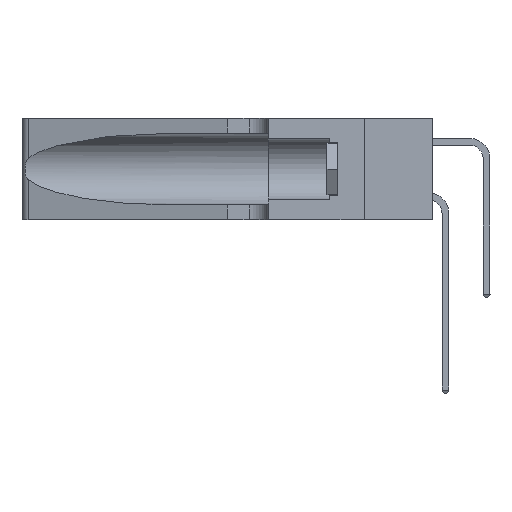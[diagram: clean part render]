
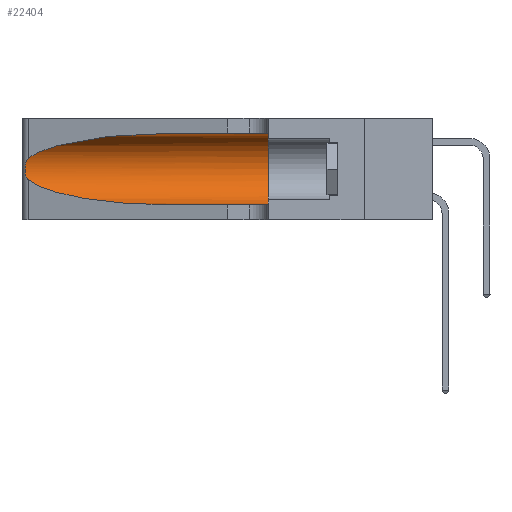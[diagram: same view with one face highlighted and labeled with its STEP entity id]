
A CAD part, left-side view. The second image highlights one B-rep face of the part: STEP entity #22404.
In plain terms, the highlighted cylindrical face has radius 3.308 mm (diameter 6.617 mm), a partial arc.
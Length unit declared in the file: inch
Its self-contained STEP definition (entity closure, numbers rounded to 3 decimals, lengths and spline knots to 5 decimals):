
#480 = CARTESIAN_POINT ( 'NONE',  ( 0.1305, 0.35, 0.05475 ) ) ;
#1663 = VECTOR ( 'NONE', #10198, 39.37008 ) ;
#1909 = CARTESIAN_POINT ( 'NONE',  ( 0.1305, 0.72297, 0.31525 ) ) ;
#1975 = CARTESIAN_POINT ( 'NONE',  ( 0.25555, 1.22993, 0.14849 ) ) ;
#2083 = ORIENTED_EDGE ( 'NONE', *, *, #28961, .T. ) ;
#4200 = CARTESIAN_POINT ( 'NONE',  ( 0.1305, 1.61858, 0.05475 ) ) ;
#4732 =( BOUNDED_CURVE ( )  B_SPLINE_CURVE ( 3, ( #27735, #27615, #33720, #15820 ),
 .UNSPECIFIED., .F., .T. ) 
 B_SPLINE_CURVE_WITH_KNOTS ( ( 4, 4 ),
 ( 1.5708, 2.84003 ),
 .UNSPECIFIED. ) 
 CURVE ( )  GEOMETRIC_REPRESENTATION_ITEM ( )  RATIONAL_B_SPLINE_CURVE ( ( 1., 0.87, 0.87, 1. ) ) 
 REPRESENTATION_ITEM ( '' )  );
#4814 = EDGE_CURVE ( 'NONE', #10529, #27757, #31335, .T. ) ;
#4888 = CARTESIAN_POINT ( 'NONE',  ( 0.25555, 1.22994, 0.2215 ) ) ;
#5431 = CARTESIAN_POINT ( 'NONE',  ( 0.25487, 1.22718, 0.14631 ) ) ;
#5658 = VERTEX_POINT ( 'NONE', #14777 ) ;
#5668 = CYLINDRICAL_SURFACE ( 'NONE', #28201, 0.13025 ) ;
#6494 = CARTESIAN_POINT ( 'NONE',  ( 0.1305, 1.61858, 0.185 ) ) ;
#7881 = CARTESIAN_POINT ( 'NONE',  ( 0.25787, 1.23484, 0.2124 ) ) ;
#9592 = CARTESIAN_POINT ( 'NONE',  ( 0.25487, 1.22718, 0.14631 ) ) ;
#9637 = LINE ( 'NONE', #4200, #1663 ) ;
#10198 = DIRECTION ( 'NONE',  ( 0., -1., 0. ) ) ;
#10529 = VERTEX_POINT ( 'NONE', #23702 ) ;
#10869 = CARTESIAN_POINT ( 'NONE',  ( 0.26018, 1.23835, 0.19895 ) ) ;
#11969 = DIRECTION ( 'NONE',  ( 0., -1., 0. ) ) ;
#13504 = DIRECTION ( 'NONE',  ( 0., 1., 0. ) ) ;
#13887 = CARTESIAN_POINT ( 'NONE',  ( 0.26075, 1.23896, 0.178 ) ) ;
#14024 = EDGE_CURVE ( 'NONE', #27757, #5658, #28487, .T. ) ;
#14453 = CARTESIAN_POINT ( 'NONE',  ( 0.1305, 0.72297, 0.05475 ) ) ;
#14777 = CARTESIAN_POINT ( 'NONE',  ( 0.1305, 0.72297, 0.05475 ) ) ;
#15820 = CARTESIAN_POINT ( 'NONE',  ( 0.25487, 1.22718, 0.22369 ) ) ;
#16603 = CARTESIAN_POINT ( 'NONE',  ( 0.1305, 0.35, 0.31525 ) ) ;
#16922 = CARTESIAN_POINT ( 'NONE',  ( 0.25856, 1.23593, 0.16098 ) ) ;
#17282 = VERTEX_POINT ( 'NONE', #1909 ) ;
#17672 = ORIENTED_EDGE ( 'NONE', *, *, #33002, .F. ) ;
#18349 = VECTOR ( 'NONE', #11969, 39.37008 ) ;
#18888 = ORIENTED_EDGE ( 'NONE', *, *, #14024, .T. ) ;
#19963 = CARTESIAN_POINT ( 'NONE',  ( 0.25639, 1.23186, 0.15144 ) ) ;
#22276 = EDGE_CURVE ( 'NONE', #17282, #31079, #35158, .T. ) ;
#22404 = ADVANCED_FACE ( 'NONE', ( #22557 ), #5668, .F. ) ;
#22557 = FACE_OUTER_BOUND ( 'NONE', #38370, .T. ) ;
#22687 = VERTEX_POINT ( 'NONE', #480 ) ;
#22972 = CARTESIAN_POINT ( 'NONE',  ( 0.25487, 1.22718, 0.14631 ) ) ;
#23365 = CARTESIAN_POINT ( 'NONE',  ( 0.2373, 1.15595, 0.08982 ) ) ;
#23702 = CARTESIAN_POINT ( 'NONE',  ( 0.25487, 1.22718, 0.22369 ) ) ;
#25795 = CARTESIAN_POINT ( 'NONE',  ( 0.25639, 1.23184, 0.21858 ) ) ;
#27376 = ORIENTED_EDGE ( 'NONE', *, *, #36530, .T. ) ;
#27615 = CARTESIAN_POINT ( 'NONE',  ( 0.18966, 0.96281, 0.31525 ) ) ;
#27735 = CARTESIAN_POINT ( 'NONE',  ( 0.1305, 0.72297, 0.31525 ) ) ;
#27757 = VERTEX_POINT ( 'NONE', #9592 ) ;
#28128 = ORIENTED_EDGE ( 'NONE', *, *, #22276, .F. ) ;
#28201 = AXIS2_PLACEMENT_3D ( 'NONE', #6494, #33424, #36457 ) ;
#28487 =( BOUNDED_CURVE ( )  B_SPLINE_CURVE ( 3, ( #5431, #23365, #32341, #14453 ),
 .UNSPECIFIED., .F., .T. ) 
 B_SPLINE_CURVE_WITH_KNOTS ( ( 4, 4 ),
 ( 3.44316, 4.71239 ),
 .UNSPECIFIED. ) 
 CURVE ( )  GEOMETRIC_REPRESENTATION_ITEM ( )  RATIONAL_B_SPLINE_CURVE ( ( 1., 0.87, 0.87, 1. ) ) 
 REPRESENTATION_ITEM ( '' )  );
#28850 = CARTESIAN_POINT ( 'NONE',  ( 0.25854, 1.2359, 0.20912 ) ) ;
#28961 = EDGE_CURVE ( 'NONE', #5658, #22687, #9637, .T. ) ;
#31079 = VERTEX_POINT ( 'NONE', #16603 ) ;
#31335 = B_SPLINE_CURVE_WITH_KNOTS ( 'NONE', 3,
 ( #34694, #4888, #25795, #7881, #28850, #10869, #31802, #13887, #34829, #16922, #37827, #19963, #1975, #22972 ),
 .UNSPECIFIED., .F., .F.,
 ( 4, 2, 2, 2, 2, 2, 4 ),
 ( 0., 0.00027, 0.00053, 0.00107, 0.0016, 0.00187, 0.00214 ),
 .UNSPECIFIED. ) ;
#31423 = CARTESIAN_POINT ( 'NONE',  ( 0.1305, 0.35, 0.185 ) ) ;
#31802 = CARTESIAN_POINT ( 'NONE',  ( 0.26075, 1.23896, 0.19203 ) ) ;
#32341 = CARTESIAN_POINT ( 'NONE',  ( 0.18966, 0.96281, 0.05475 ) ) ;
#32902 = CARTESIAN_POINT ( 'NONE',  ( 0.1305, 1.61858, 0.31525 ) ) ;
#33002 = EDGE_CURVE ( 'NONE', #31079, #22687, #36838, .T. ) ;
#33424 = DIRECTION ( 'NONE',  ( 0., -1., 0. ) ) ;
#33684 = AXIS2_PLACEMENT_3D ( 'NONE', #31423, #13504, #34433 ) ;
#33720 = CARTESIAN_POINT ( 'NONE',  ( 0.2373, 1.15595, 0.28018 ) ) ;
#34433 = DIRECTION ( 'NONE',  ( 0., 0., 1. ) ) ;
#34694 = CARTESIAN_POINT ( 'NONE',  ( 0.25487, 1.22718, 0.22369 ) ) ;
#34829 = CARTESIAN_POINT ( 'NONE',  ( 0.26017, 1.23833, 0.17102 ) ) ;
#35158 = LINE ( 'NONE', #32902, #18349 ) ;
#36457 = DIRECTION ( 'NONE',  ( 0., 0., -1. ) ) ;
#36530 = EDGE_CURVE ( 'NONE', #17282, #10529, #4732, .T. ) ;
#36838 = CIRCLE ( 'NONE', #33684, 0.13025 ) ;
#36934 = ORIENTED_EDGE ( 'NONE', *, *, #4814, .T. ) ;
#37827 = CARTESIAN_POINT ( 'NONE',  ( 0.25789, 1.23486, 0.15765 ) ) ;
#38370 = EDGE_LOOP ( 'NONE', ( #27376, #36934, #18888, #2083, #17672, #28128 ) ) ;
